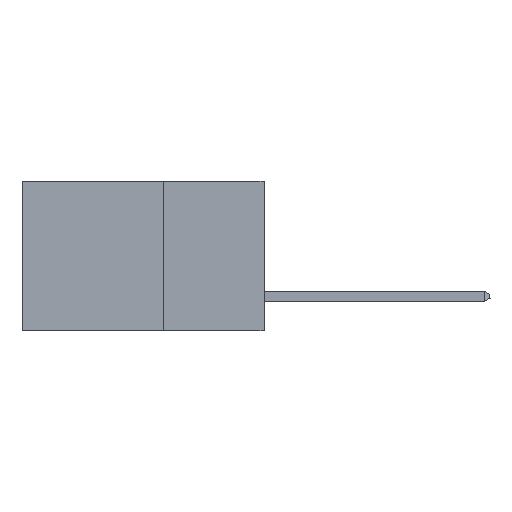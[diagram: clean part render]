
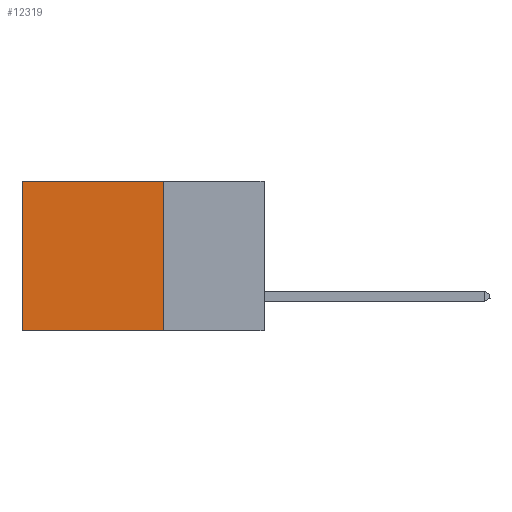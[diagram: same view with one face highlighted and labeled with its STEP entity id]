
A CAD part, left-side view. The second image highlights one B-rep face of the part: STEP entity #12319.
In plain terms, the highlighted planar face has unit normal (-1, 0, 0).
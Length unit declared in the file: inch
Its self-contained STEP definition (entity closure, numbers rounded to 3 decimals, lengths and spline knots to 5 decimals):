
#130 = LINE ( 'NONE', #1024, #11393 ) ;
#263 = EDGE_CURVE ( 'NONE', #3546, #12766, #130, .T. ) ;
#560 = ORIENTED_EDGE ( 'NONE', *, *, #1729, .T. ) ;
#1024 = CARTESIAN_POINT ( 'NONE',  ( 0.298, 0.25, -0.37 ) ) ;
#1515 = LINE ( 'NONE', #6786, #6926 ) ;
#1520 = DIRECTION ( 'NONE',  ( 0., 0., -1. ) ) ;
#1729 = EDGE_CURVE ( 'NONE', #8490, #12766, #11342, .T. ) ;
#1906 = DIRECTION ( 'NONE',  ( 0., 0., -1. ) ) ;
#2340 = ORIENTED_EDGE ( 'NONE', *, *, #263, .F. ) ;
#2566 = CARTESIAN_POINT ( 'NONE',  ( 0.298, 0.6, 0. ) ) ;
#2828 = CARTESIAN_POINT ( 'NONE',  ( 0.298, 0.25, -0.37 ) ) ;
#3546 = VERTEX_POINT ( 'NONE', #2828 ) ;
#4140 = CARTESIAN_POINT ( 'NONE',  ( 0.298, 0.25, 0. ) ) ;
#4276 = LINE ( 'NONE', #4140, #11369 ) ;
#5612 = ORIENTED_EDGE ( 'NONE', *, *, #6360, .F. ) ;
#5691 = CARTESIAN_POINT ( 'NONE',  ( 0.298, 0.25, 0. ) ) ;
#5942 = FACE_OUTER_BOUND ( 'NONE', #9195, .T. ) ;
#5996 = DIRECTION ( 'NONE',  ( 0., 0., -1. ) ) ;
#6162 = DIRECTION ( 'NONE',  ( 0., 1., 0. ) ) ;
#6360 = EDGE_CURVE ( 'NONE', #8237, #3546, #4276, .T. ) ;
#6555 = CARTESIAN_POINT ( 'NONE',  ( 0.298, 0.6, -0.37 ) ) ;
#6786 = CARTESIAN_POINT ( 'NONE',  ( 0.298, 0.25, 0. ) ) ;
#6926 = VECTOR ( 'NONE', #6162, 39.37008 ) ;
#7354 = ORIENTED_EDGE ( 'NONE', *, *, #9523, .T. ) ;
#7825 = CARTESIAN_POINT ( 'NONE',  ( 0.298, 0.25, 0. ) ) ;
#8039 = AXIS2_PLACEMENT_3D ( 'NONE', #7825, #12660, #1906 ) ;
#8237 = VERTEX_POINT ( 'NONE', #5691 ) ;
#8297 = VECTOR ( 'NONE', #1520, 39.37008 ) ;
#8490 = VERTEX_POINT ( 'NONE', #10336 ) ;
#8714 = PLANE ( 'NONE',  #8039 ) ;
#8935 = DIRECTION ( 'NONE',  ( 0., 1., 0. ) ) ;
#9195 = EDGE_LOOP ( 'NONE', ( #560, #2340, #5612, #7354 ) ) ;
#9523 = EDGE_CURVE ( 'NONE', #8237, #8490, #1515, .T. ) ;
#10336 = CARTESIAN_POINT ( 'NONE',  ( 0.298, 0.6, 0. ) ) ;
#11342 = LINE ( 'NONE', #2566, #8297 ) ;
#11369 = VECTOR ( 'NONE', #5996, 39.37008 ) ;
#11393 = VECTOR ( 'NONE', #8935, 39.37008 ) ;
#12319 = ADVANCED_FACE ( 'NONE', ( #5942 ), #8714, .F. ) ;
#12660 = DIRECTION ( 'NONE',  ( 1., 0., 0. ) ) ;
#12766 = VERTEX_POINT ( 'NONE', #6555 ) ;
